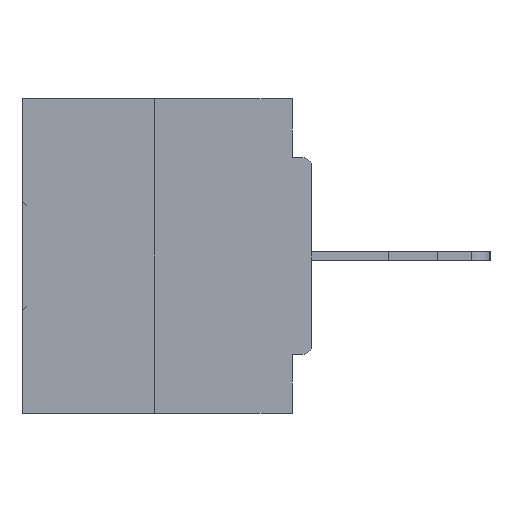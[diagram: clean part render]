
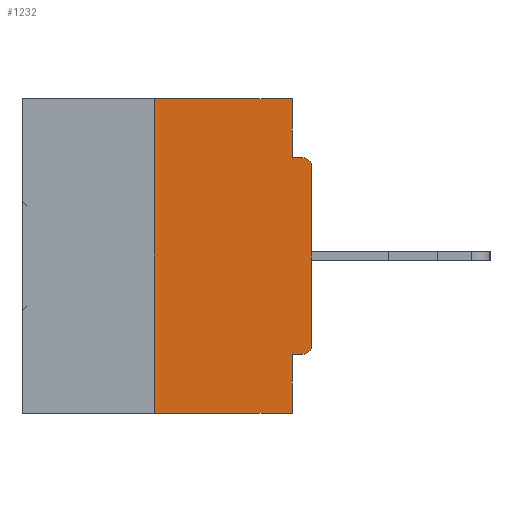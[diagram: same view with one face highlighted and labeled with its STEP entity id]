
A CAD part, left-side view. The second image highlights one B-rep face of the part: STEP entity #1232.
In plain terms, the highlighted planar face has unit normal (-1, 0, 0).
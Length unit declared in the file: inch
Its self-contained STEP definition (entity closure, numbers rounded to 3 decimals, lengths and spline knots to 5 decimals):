
#143 = CARTESIAN_POINT ( 'NONE',  ( 0., 0.031, 0. ) ) ;
#415 = AXIS2_PLACEMENT_3D ( 'NONE', #24480, #21467, #33779 ) ;
#1232 = ADVANCED_FACE ( 'NONE', ( #19745 ), #13908, .F. ) ;
#1310 = EDGE_CURVE ( 'NONE', #33533, #39069, #39248, .T. ) ;
#1629 = LINE ( 'NONE', #4642, #30304 ) ;
#1796 = ORIENTED_EDGE ( 'NONE', *, *, #4034, .F. ) ;
#1816 = VECTOR ( 'NONE', #34559, 39.37008 ) ;
#2412 = VECTOR ( 'NONE', #11888, 39.37008 ) ;
#3730 = ORIENTED_EDGE ( 'NONE', *, *, #25989, .T. ) ;
#4034 = EDGE_CURVE ( 'NONE', #15004, #33053, #11742, .T. ) ;
#4182 = VECTOR ( 'NONE', #13840, 39.37008 ) ;
#4642 = CARTESIAN_POINT ( 'NONE',  ( 0., 0.031, 0. ) ) ;
#4681 = DIRECTION ( 'NONE',  ( 0., 0., -1. ) ) ;
#5363 = EDGE_CURVE ( 'NONE', #25795, #10609, #14159, .T. ) ;
#5489 = ORIENTED_EDGE ( 'NONE', *, *, #30347, .F. ) ;
#6027 = DIRECTION ( 'NONE',  ( 0., 0., -1. ) ) ;
#6605 = LINE ( 'NONE', #30757, #1816 ) ;
#7193 = EDGE_CURVE ( 'NONE', #12338, #15355, #1629, .T. ) ;
#7472 = DIRECTION ( 'NONE',  ( 0., 0., -1. ) ) ;
#8842 = CARTESIAN_POINT ( 'NONE',  ( 0., 0.031, -0.5 ) ) ;
#10609 = VERTEX_POINT ( 'NONE', #27132 ) ;
#11170 = CARTESIAN_POINT ( 'NONE',  ( 0., 0., -0.4065 ) ) ;
#11187 = ORIENTED_EDGE ( 'NONE', *, *, #31298, .F. ) ;
#11418 = AXIS2_PLACEMENT_3D ( 'NONE', #32054, #29023, #4681 ) ;
#11742 = LINE ( 'NONE', #14550, #30989 ) ;
#11888 = DIRECTION ( 'NONE',  ( 0., 0., 1. ) ) ;
#12338 = VERTEX_POINT ( 'NONE', #143 ) ;
#13203 = CARTESIAN_POINT ( 'NONE',  ( 0., 0., -0.1085 ) ) ;
#13704 = ORIENTED_EDGE ( 'NONE', *, *, #1310, .T. ) ;
#13840 = DIRECTION ( 'NONE',  ( 0., -1., 0. ) ) ;
#13908 = PLANE ( 'NONE',  #11418 ) ;
#14159 = LINE ( 'NONE', #11170, #22652 ) ;
#14440 = LINE ( 'NONE', #29166, #4182 ) ;
#14550 = CARTESIAN_POINT ( 'NONE',  ( 0., 0.25, 0. ) ) ;
#15004 = VERTEX_POINT ( 'NONE', #38011 ) ;
#15355 = VERTEX_POINT ( 'NONE', #27133 ) ;
#15643 = EDGE_LOOP ( 'NONE', ( #5489, #1796, #3730, #11187, #30492, #19118, #13704, #25251, #24068, #29665 ) ) ;
#16429 = CARTESIAN_POINT ( 'NONE',  ( 0., 0., -0.0935 ) ) ;
#18106 = EDGE_CURVE ( 'NONE', #25795, #33533, #39588, .T. ) ;
#19011 = CIRCLE ( 'NONE', #415, 0.015 ) ;
#19118 = ORIENTED_EDGE ( 'NONE', *, *, #18106, .T. ) ;
#19745 = FACE_OUTER_BOUND ( 'NONE', #15643, .T. ) ;
#21143 = EDGE_CURVE ( 'NONE', #15355, #21695, #22902, .T. ) ;
#21467 = DIRECTION ( 'NONE',  ( -1., 0., 0. ) ) ;
#21695 = VERTEX_POINT ( 'NONE', #36336 ) ;
#22235 = AXIS2_PLACEMENT_3D ( 'NONE', #38341, #23447, #23043 ) ;
#22652 = VECTOR ( 'NONE', #38718, 39.37008 ) ;
#22737 = CARTESIAN_POINT ( 'NONE',  ( 0., 0.031, -0.5 ) ) ;
#22902 = LINE ( 'NONE', #16429, #30747 ) ;
#23043 = DIRECTION ( 'NONE',  ( 0., 0., -1. ) ) ;
#23447 = DIRECTION ( 'NONE',  ( -1., 0., 0. ) ) ;
#24068 = ORIENTED_EDGE ( 'NONE', *, *, #21143, .F. ) ;
#24193 = VERTEX_POINT ( 'NONE', #22737 ) ;
#24480 = CARTESIAN_POINT ( 'NONE',  ( 0., 0.015, -0.1085 ) ) ;
#25251 = ORIENTED_EDGE ( 'NONE', *, *, #29095, .T. ) ;
#25795 = VERTEX_POINT ( 'NONE', #39677 ) ;
#25989 = EDGE_CURVE ( 'NONE', #15004, #24193, #14440, .T. ) ;
#27052 = DIRECTION ( 'NONE',  ( 0., 0., 1. ) ) ;
#27132 = CARTESIAN_POINT ( 'NONE',  ( 0., 0.031, -0.4065 ) ) ;
#27133 = CARTESIAN_POINT ( 'NONE',  ( 0., 0.031, -0.0935 ) ) ;
#29023 = DIRECTION ( 'NONE',  ( 1., 0., 0. ) ) ;
#29095 = EDGE_CURVE ( 'NONE', #39069, #21695, #19011, .T. ) ;
#29166 = CARTESIAN_POINT ( 'NONE',  ( 0., 0.46, -0.5 ) ) ;
#29487 = VECTOR ( 'NONE', #6027, 39.37008 ) ;
#29665 = ORIENTED_EDGE ( 'NONE', *, *, #7193, .F. ) ;
#29834 = CARTESIAN_POINT ( 'NONE',  ( 0., 0., 0. ) ) ;
#30304 = VECTOR ( 'NONE', #7472, 39.37008 ) ;
#30347 = EDGE_CURVE ( 'NONE', #33053, #12338, #6605, .T. ) ;
#30492 = ORIENTED_EDGE ( 'NONE', *, *, #5363, .F. ) ;
#30747 = VECTOR ( 'NONE', #35209, 39.37008 ) ;
#30757 = CARTESIAN_POINT ( 'NONE',  ( 0., 0.46, 0. ) ) ;
#30989 = VECTOR ( 'NONE', #27052, 39.37008 ) ;
#31298 = EDGE_CURVE ( 'NONE', #10609, #24193, #39384, .T. ) ;
#32054 = CARTESIAN_POINT ( 'NONE',  ( 0., 0.46, 0. ) ) ;
#32875 = CARTESIAN_POINT ( 'NONE',  ( 0., 0., -0.3915 ) ) ;
#33053 = VERTEX_POINT ( 'NONE', #33314 ) ;
#33314 = CARTESIAN_POINT ( 'NONE',  ( 0., 0.25, 0. ) ) ;
#33533 = VERTEX_POINT ( 'NONE', #32875 ) ;
#33779 = DIRECTION ( 'NONE',  ( 0., 0., -1. ) ) ;
#34559 = DIRECTION ( 'NONE',  ( 0., -1., 0. ) ) ;
#35209 = DIRECTION ( 'NONE',  ( 0., -1., 0. ) ) ;
#36336 = CARTESIAN_POINT ( 'NONE',  ( 0., 0.015, -0.0935 ) ) ;
#38011 = CARTESIAN_POINT ( 'NONE',  ( 0., 0.25, -0.5 ) ) ;
#38341 = CARTESIAN_POINT ( 'NONE',  ( 0., 0.015, -0.3915 ) ) ;
#38718 = DIRECTION ( 'NONE',  ( 0., 1., 0. ) ) ;
#39069 = VERTEX_POINT ( 'NONE', #13203 ) ;
#39248 = LINE ( 'NONE', #29834, #2412 ) ;
#39384 = LINE ( 'NONE', #8842, #29487 ) ;
#39588 = CIRCLE ( 'NONE', #22235, 0.015 ) ;
#39677 = CARTESIAN_POINT ( 'NONE',  ( 0., 0.015, -0.4065 ) ) ;
